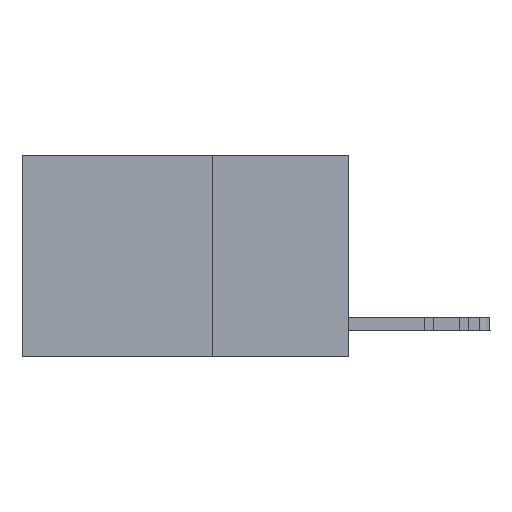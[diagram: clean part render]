
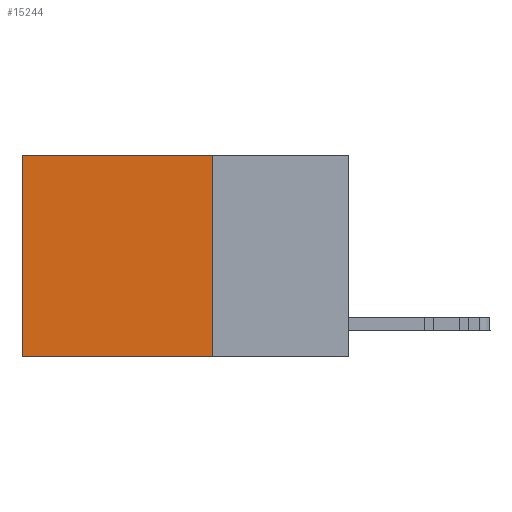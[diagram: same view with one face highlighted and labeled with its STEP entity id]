
A CAD part, left-side view. The second image highlights one B-rep face of the part: STEP entity #15244.
In plain terms, the highlighted planar face has unit normal (-1, 0, 0).
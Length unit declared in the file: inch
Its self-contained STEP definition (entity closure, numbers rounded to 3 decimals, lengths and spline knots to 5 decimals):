
#370 = CARTESIAN_POINT ( 'NONE',  ( 0.2625, 0.6, 0. ) ) ;
#732 = DIRECTION ( 'NONE',  ( 0., 0., -1. ) ) ;
#1311 = FACE_OUTER_BOUND ( 'NONE', #7715, .T. ) ;
#1457 = DIRECTION ( 'NONE',  ( 1., 0., 0. ) ) ;
#2499 = ORIENTED_EDGE ( 'NONE', *, *, #25537, .F. ) ;
#2611 = VERTEX_POINT ( 'NONE', #370 ) ;
#3604 = CARTESIAN_POINT ( 'NONE',  ( 0.2625, 0.25, 0. ) ) ;
#4622 = VECTOR ( 'NONE', #13650, 39.37008 ) ;
#4970 = EDGE_CURVE ( 'NONE', #2611, #9365, #15828, .T. ) ;
#5160 = CARTESIAN_POINT ( 'NONE',  ( 0.2625, 0.25, 0. ) ) ;
#6680 = CARTESIAN_POINT ( 'NONE',  ( 0.2625, 0.25, -0.37 ) ) ;
#7293 = EDGE_CURVE ( 'NONE', #14113, #2611, #25208, .T. ) ;
#7715 = EDGE_LOOP ( 'NONE', ( #10760, #2499, #15838, #20375 ) ) ;
#8071 = CARTESIAN_POINT ( 'NONE',  ( 0.2625, 0.25, 0. ) ) ;
#9308 = DIRECTION ( 'NONE',  ( 0., 1., 0. ) ) ;
#9365 = VERTEX_POINT ( 'NONE', #25139 ) ;
#9761 = EDGE_CURVE ( 'NONE', #14113, #12005, #20005, .T. ) ;
#9818 = DIRECTION ( 'NONE',  ( 0., 0., -1. ) ) ;
#10760 = ORIENTED_EDGE ( 'NONE', *, *, #4970, .T. ) ;
#12005 = VERTEX_POINT ( 'NONE', #26065 ) ;
#13650 = DIRECTION ( 'NONE',  ( 0., 1., 0. ) ) ;
#13695 = DIRECTION ( 'NONE',  ( 0., 0., -1. ) ) ;
#14113 = VERTEX_POINT ( 'NONE', #3604 ) ;
#15244 = ADVANCED_FACE ( 'NONE', ( #1311 ), #25766, .F. ) ;
#15828 = LINE ( 'NONE', #20519, #27342 ) ;
#15838 = ORIENTED_EDGE ( 'NONE', *, *, #9761, .F. ) ;
#18309 = AXIS2_PLACEMENT_3D ( 'NONE', #8071, #1457, #9818 ) ;
#20005 = LINE ( 'NONE', #27037, #28626 ) ;
#20375 = ORIENTED_EDGE ( 'NONE', *, *, #7293, .T. ) ;
#20519 = CARTESIAN_POINT ( 'NONE',  ( 0.2625, 0.6, 0. ) ) ;
#22736 = LINE ( 'NONE', #6680, #23170 ) ;
#23170 = VECTOR ( 'NONE', #9308, 39.37008 ) ;
#25139 = CARTESIAN_POINT ( 'NONE',  ( 0.2625, 0.6, -0.37 ) ) ;
#25208 = LINE ( 'NONE', #5160, #4622 ) ;
#25537 = EDGE_CURVE ( 'NONE', #12005, #9365, #22736, .T. ) ;
#25766 = PLANE ( 'NONE',  #18309 ) ;
#26065 = CARTESIAN_POINT ( 'NONE',  ( 0.2625, 0.25, -0.37 ) ) ;
#27037 = CARTESIAN_POINT ( 'NONE',  ( 0.2625, 0.25, 0. ) ) ;
#27342 = VECTOR ( 'NONE', #732, 39.37008 ) ;
#28626 = VECTOR ( 'NONE', #13695, 39.37008 ) ;
